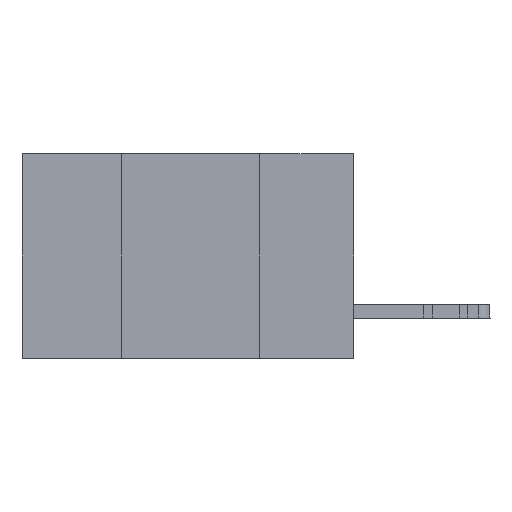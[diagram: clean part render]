
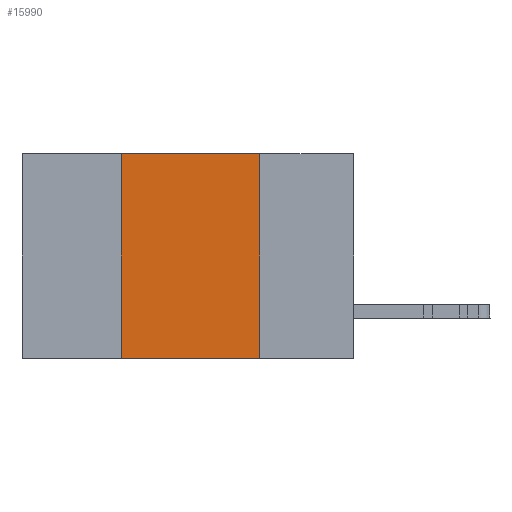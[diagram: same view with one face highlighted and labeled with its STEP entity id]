
A CAD part, left-side view. The second image highlights one B-rep face of the part: STEP entity #15990.
In plain terms, the highlighted planar face has unit normal (-1, 0, 0).
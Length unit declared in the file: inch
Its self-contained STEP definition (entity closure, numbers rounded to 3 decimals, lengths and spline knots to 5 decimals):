
#1356 = CARTESIAN_POINT ( 'NONE',  ( 0., 0.42, 0. ) ) ;
#3330 = EDGE_CURVE ( 'NONE', #36441, #35504, #4549, .T. ) ;
#3517 = CARTESIAN_POINT ( 'NONE',  ( 0., 0.17, 0. ) ) ;
#4549 = LINE ( 'NONE', #1356, #38233 ) ;
#6195 = CARTESIAN_POINT ( 'NONE',  ( 0., 0.6, 0. ) ) ;
#6768 = DIRECTION ( 'NONE',  ( 0., -1., 0. ) ) ;
#7618 = LINE ( 'NONE', #3517, #23037 ) ;
#7871 = DIRECTION ( 'NONE',  ( 0., 0., 1. ) ) ;
#8487 = ORIENTED_EDGE ( 'NONE', *, *, #27152, .T. ) ;
#10136 = LINE ( 'NONE', #6195, #20921 ) ;
#10324 = CARTESIAN_POINT ( 'NONE',  ( 0., 0.42, -0.37 ) ) ;
#15990 = ADVANCED_FACE ( 'NONE', ( #26856 ), #36404, .F. ) ;
#16699 = ORIENTED_EDGE ( 'NONE', *, *, #22479, .F. ) ;
#16948 = CARTESIAN_POINT ( 'NONE',  ( 0., 0.6, 0. ) ) ;
#19990 = DIRECTION ( 'NONE',  ( 0., 0., -1. ) ) ;
#20277 = DIRECTION ( 'NONE',  ( 1., 0., 0. ) ) ;
#20921 = VECTOR ( 'NONE', #29081, 39.37008 ) ;
#21900 = EDGE_CURVE ( 'NONE', #25801, #31141, #7618, .T. ) ;
#22479 = EDGE_CURVE ( 'NONE', #35504, #25801, #10136, .T. ) ;
#23037 = VECTOR ( 'NONE', #19990, 39.37008 ) ;
#23125 = VECTOR ( 'NONE', #6768, 39.37008 ) ;
#25369 = CARTESIAN_POINT ( 'NONE',  ( 0., 0.42, 0. ) ) ;
#25573 = CARTESIAN_POINT ( 'NONE',  ( 0., 0.17, 0. ) ) ;
#25801 = VERTEX_POINT ( 'NONE', #25573 ) ;
#26418 = CARTESIAN_POINT ( 'NONE',  ( 0., 0.6, -0.37 ) ) ;
#26856 = FACE_OUTER_BOUND ( 'NONE', #33124, .T. ) ;
#27152 = EDGE_CURVE ( 'NONE', #36441, #31141, #31685, .T. ) ;
#28945 = ORIENTED_EDGE ( 'NONE', *, *, #3330, .F. ) ;
#29081 = DIRECTION ( 'NONE',  ( 0., -1., 0. ) ) ;
#29309 = AXIS2_PLACEMENT_3D ( 'NONE', #16948, #20277, #29375 ) ;
#29375 = DIRECTION ( 'NONE',  ( 0., 0., -1. ) ) ;
#31141 = VERTEX_POINT ( 'NONE', #35782 ) ;
#31685 = LINE ( 'NONE', #26418, #23125 ) ;
#33124 = EDGE_LOOP ( 'NONE', ( #38182, #16699, #28945, #8487 ) ) ;
#35504 = VERTEX_POINT ( 'NONE', #25369 ) ;
#35782 = CARTESIAN_POINT ( 'NONE',  ( 0., 0.17, -0.37 ) ) ;
#36404 = PLANE ( 'NONE',  #29309 ) ;
#36441 = VERTEX_POINT ( 'NONE', #10324 ) ;
#38182 = ORIENTED_EDGE ( 'NONE', *, *, #21900, .F. ) ;
#38233 = VECTOR ( 'NONE', #7871, 39.37008 ) ;
